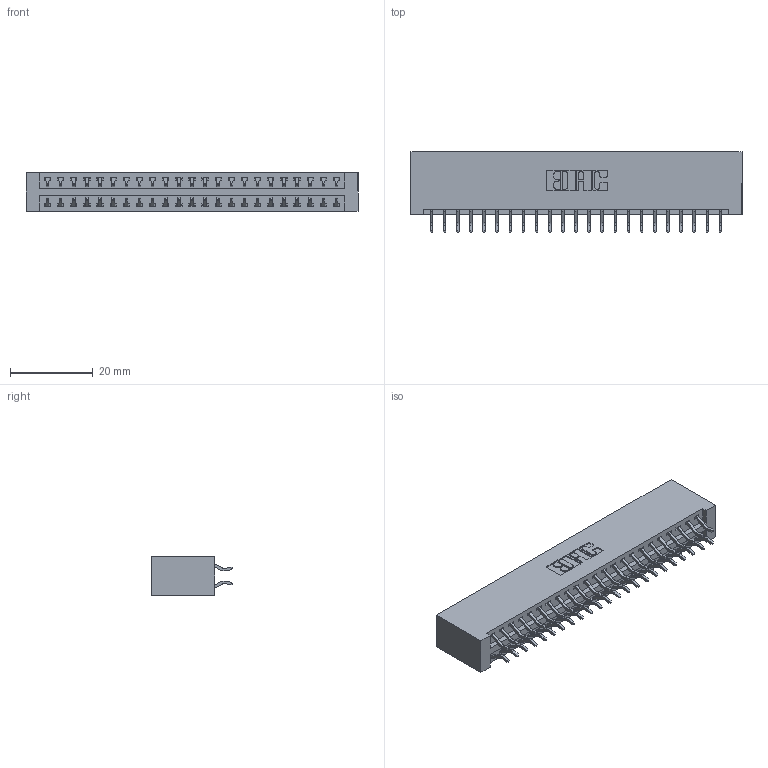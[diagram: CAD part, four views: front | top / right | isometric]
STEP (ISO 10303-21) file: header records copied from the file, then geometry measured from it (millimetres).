
FILE_DESCRIPTION (( 'STEP AP203' ), '1' );
FILE_NAME ('346-046-556-201.STEP', '2018-08-25T06:17:58', ( '' ), ( '' ), 'SwSTEP 2.0', 'SolidWorks 2016', '' );
FILE_SCHEMA (( 'CONFIG_CONTROL_DESIGN' ));
Length unit declared in the file: inch
Products named in the file (3): 346 Part_No Mounting Lugs; 345-292-001_556 Tail; 346-046-556-201
Assembly tree (47 placements, depth 2):
  346-046-556-201
    346 Part_No Mounting Lugs
    345-292-001_556 Tail  x46
Bounding box: 80.26 x 19.57 x 9.4 mm (x, y, z)
Volume: 8250.6 mm3; surface area: 11162.9 mm2
Topology: 47 solids, 47 shells, 2782 faces, 8263 edges, 5446 vertices
Faces by surface type: plane 1866, cylinder 916
Entity records: 17511 total; most frequent: CARTESIAN_POINT 2924, ORIENTED_EDGE 2846, DIRECTION 2611, EDGE_CURVE 1423, VECTOR 1199, LINE 1199, VERTEX_POINT 946, AXIS2_PLACEMENT_3D 706
